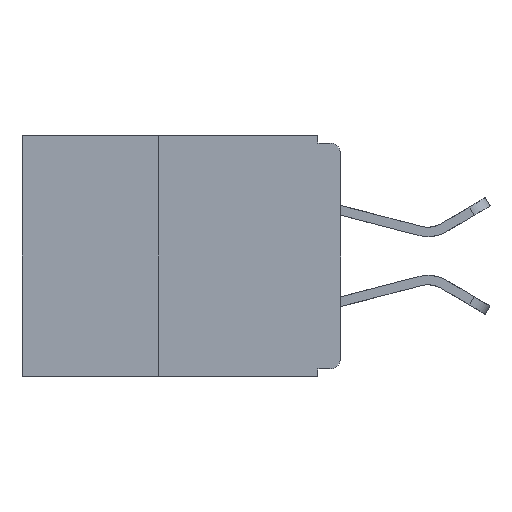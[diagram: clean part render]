
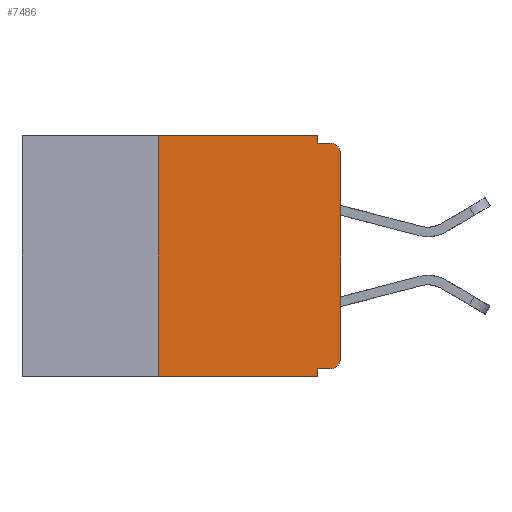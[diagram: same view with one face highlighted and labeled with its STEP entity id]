
A CAD part, left-side view. The second image highlights one B-rep face of the part: STEP entity #7486.
In plain terms, the highlighted planar face has unit normal (-1, 0, 0).
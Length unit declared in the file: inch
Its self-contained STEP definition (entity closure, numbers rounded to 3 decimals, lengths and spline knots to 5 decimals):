
#206 = ORIENTED_EDGE ( 'NONE', *, *, #3646, .F. ) ;
#218 = ORIENTED_EDGE ( 'NONE', *, *, #3335, .F. ) ;
#239 = LINE ( 'NONE', #11033, #2498 ) ;
#260 = CARTESIAN_POINT ( 'NONE',  ( 0., 0.25, -0.33 ) ) ;
#313 = DIRECTION ( 'NONE',  ( 0., -1., 0. ) ) ;
#782 = CARTESIAN_POINT ( 'NONE',  ( 0., 0.25, 0. ) ) ;
#933 = CARTESIAN_POINT ( 'NONE',  ( 0., 0., -0.025 ) ) ;
#998 = DIRECTION ( 'NONE',  ( 0., -1., 0. ) ) ;
#1008 = VECTOR ( 'NONE', #7555, 39.37008 ) ;
#1348 = VERTEX_POINT ( 'NONE', #10058 ) ;
#1599 = EDGE_CURVE ( 'NONE', #3555, #7607, #3938, .T. ) ;
#1736 = ORIENTED_EDGE ( 'NONE', *, *, #3589, .T. ) ;
#1803 = VECTOR ( 'NONE', #5914, 39.37008 ) ;
#1901 = FACE_OUTER_BOUND ( 'NONE', #12452, .T. ) ;
#2498 = VECTOR ( 'NONE', #3438, 39.37008 ) ;
#2599 = ORIENTED_EDGE ( 'NONE', *, *, #1599, .F. ) ;
#2801 = VECTOR ( 'NONE', #4431, 39.37008 ) ;
#3013 = DIRECTION ( 'NONE',  ( 0., 0., -1. ) ) ;
#3203 = CARTESIAN_POINT ( 'NONE',  ( 0., 0.031, -0.33 ) ) ;
#3225 = EDGE_CURVE ( 'NONE', #8327, #13511, #8994, .T. ) ;
#3335 = EDGE_CURVE ( 'NONE', #12950, #8086, #9857, .T. ) ;
#3438 = DIRECTION ( 'NONE',  ( 0., -1., 0. ) ) ;
#3555 = VERTEX_POINT ( 'NONE', #12326 ) ;
#3570 = ORIENTED_EDGE ( 'NONE', *, *, #4028, .F. ) ;
#3589 = EDGE_CURVE ( 'NONE', #13511, #13960, #12514, .T. ) ;
#3646 = EDGE_CURVE ( 'NONE', #8327, #3555, #5691, .T. ) ;
#3647 = CARTESIAN_POINT ( 'NONE',  ( 0., 0.25, -0.33 ) ) ;
#3714 = VERTEX_POINT ( 'NONE', #6763 ) ;
#3764 = ORIENTED_EDGE ( 'NONE', *, *, #13686, .F. ) ;
#3895 = ORIENTED_EDGE ( 'NONE', *, *, #3225, .T. ) ;
#3938 = LINE ( 'NONE', #11239, #1008 ) ;
#4028 = EDGE_CURVE ( 'NONE', #8086, #1348, #10011, .T. ) ;
#4304 = DIRECTION ( 'NONE',  ( 0., 0., -1. ) ) ;
#4431 = DIRECTION ( 'NONE',  ( 0., 1., 0. ) ) ;
#4504 = VERTEX_POINT ( 'NONE', #9814 ) ;
#4506 = CARTESIAN_POINT ( 'NONE',  ( 0., 0.437, 0. ) ) ;
#4831 = CARTESIAN_POINT ( 'NONE',  ( 0., 0.031, 0. ) ) ;
#5144 = EDGE_CURVE ( 'NONE', #13960, #4504, #6714, .T. ) ;
#5163 = PLANE ( 'NONE',  #7198 ) ;
#5212 = DIRECTION ( 'NONE',  ( 0., 0., 1. ) ) ;
#5342 = AXIS2_PLACEMENT_3D ( 'NONE', #11954, #11935, #11892 ) ;
#5610 = ORIENTED_EDGE ( 'NONE', *, *, #9524, .F. ) ;
#5691 = LINE ( 'NONE', #10931, #2801 ) ;
#5914 = DIRECTION ( 'NONE',  ( 0., 0., -1. ) ) ;
#6294 = VECTOR ( 'NONE', #313, 39.37008 ) ;
#6519 = CARTESIAN_POINT ( 'NONE',  ( 0., 0.015, -0.305 ) ) ;
#6714 = CIRCLE ( 'NONE', #5342, 0.015 ) ;
#6763 = CARTESIAN_POINT ( 'NONE',  ( 0., 0.031, -0.01 ) ) ;
#6785 = VECTOR ( 'NONE', #8528, 39.37008 ) ;
#6957 = VECTOR ( 'NONE', #5212, 39.37008 ) ;
#7198 = AXIS2_PLACEMENT_3D ( 'NONE', #8429, #9551, #3013 ) ;
#7486 = ADVANCED_FACE ( 'NONE', ( #1901 ), #5163, .F. ) ;
#7555 = DIRECTION ( 'NONE',  ( 0., 0., -1. ) ) ;
#7607 = VERTEX_POINT ( 'NONE', #3203 ) ;
#7924 = CARTESIAN_POINT ( 'NONE',  ( 0., 0.437, -0.33 ) ) ;
#8086 = VERTEX_POINT ( 'NONE', #782 ) ;
#8327 = VERTEX_POINT ( 'NONE', #12081 ) ;
#8425 = EDGE_CURVE ( 'NONE', #12950, #7607, #9176, .T. ) ;
#8429 = CARTESIAN_POINT ( 'NONE',  ( 0., 0.437, 0. ) ) ;
#8528 = DIRECTION ( 'NONE',  ( 0., 0., 1. ) ) ;
#8735 = CARTESIAN_POINT ( 'NONE',  ( 0., 0., 0. ) ) ;
#8994 = CIRCLE ( 'NONE', #9435, 0.015 ) ;
#9176 = LINE ( 'NONE', #7924, #6294 ) ;
#9435 = AXIS2_PLACEMENT_3D ( 'NONE', #6519, #9564, #4304 ) ;
#9522 = ORIENTED_EDGE ( 'NONE', *, *, #8425, .T. ) ;
#9524 = EDGE_CURVE ( 'NONE', #3714, #4504, #239, .T. ) ;
#9551 = DIRECTION ( 'NONE',  ( 1., 0., 0. ) ) ;
#9564 = DIRECTION ( 'NONE',  ( -1., 0., 0. ) ) ;
#9665 = VECTOR ( 'NONE', #998, 39.37008 ) ;
#9814 = CARTESIAN_POINT ( 'NONE',  ( 0., 0.015, -0.01 ) ) ;
#9857 = LINE ( 'NONE', #3647, #6957 ) ;
#10011 = LINE ( 'NONE', #4506, #9665 ) ;
#10058 = CARTESIAN_POINT ( 'NONE',  ( 0., 0.031, 0. ) ) ;
#10931 = CARTESIAN_POINT ( 'NONE',  ( 0., 0., -0.32 ) ) ;
#11033 = CARTESIAN_POINT ( 'NONE',  ( 0., 0., -0.01 ) ) ;
#11239 = CARTESIAN_POINT ( 'NONE',  ( 0., 0.031, -0.33 ) ) ;
#11892 = DIRECTION ( 'NONE',  ( 0., 0., -1. ) ) ;
#11935 = DIRECTION ( 'NONE',  ( -1., 0., 0. ) ) ;
#11954 = CARTESIAN_POINT ( 'NONE',  ( 0., 0.015, -0.025 ) ) ;
#12081 = CARTESIAN_POINT ( 'NONE',  ( 0., 0.015, -0.32 ) ) ;
#12326 = CARTESIAN_POINT ( 'NONE',  ( 0., 0.031, -0.32 ) ) ;
#12452 = EDGE_LOOP ( 'NONE', ( #1736, #12669, #5610, #3764, #3570, #218, #9522, #2599, #206, #3895 ) ) ;
#12514 = LINE ( 'NONE', #8735, #6785 ) ;
#12669 = ORIENTED_EDGE ( 'NONE', *, *, #5144, .T. ) ;
#12950 = VERTEX_POINT ( 'NONE', #260 ) ;
#13092 = CARTESIAN_POINT ( 'NONE',  ( 0., 0., -0.305 ) ) ;
#13271 = LINE ( 'NONE', #4831, #1803 ) ;
#13511 = VERTEX_POINT ( 'NONE', #13092 ) ;
#13686 = EDGE_CURVE ( 'NONE', #1348, #3714, #13271, .T. ) ;
#13960 = VERTEX_POINT ( 'NONE', #933 ) ;
